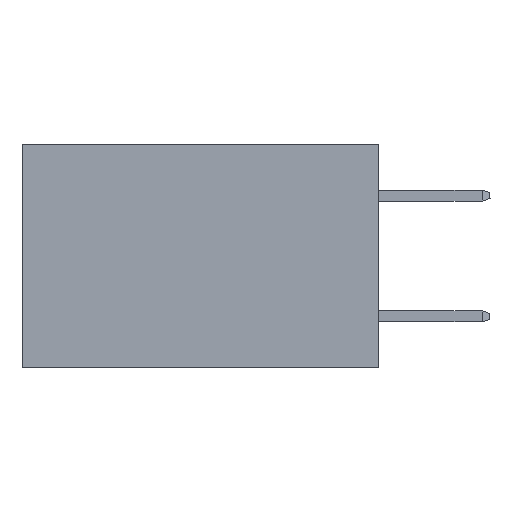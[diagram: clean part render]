
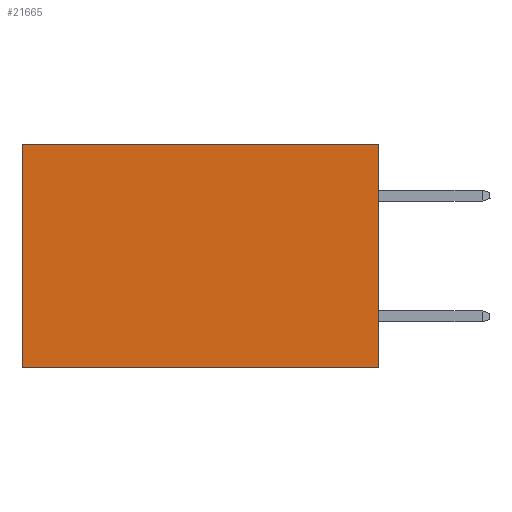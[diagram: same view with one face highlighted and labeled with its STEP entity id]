
A CAD part, left-side view. The second image highlights one B-rep face of the part: STEP entity #21665.
In plain terms, the highlighted planar face has unit normal (-1, 0, 0).
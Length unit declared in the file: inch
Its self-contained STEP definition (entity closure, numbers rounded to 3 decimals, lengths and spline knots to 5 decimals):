
#266 = VECTOR ( 'NONE', #4841, 39.37008 ) ;
#734 = AXIS2_PLACEMENT_3D ( 'NONE', #18859, #20709, #9584 ) ;
#857 = LINE ( 'NONE', #14212, #266 ) ;
#997 = CARTESIAN_POINT ( 'NONE',  ( 0.277, 0.59, 0. ) ) ;
#1750 = EDGE_CURVE ( 'NONE', #14072, #23244, #3507, .T. ) ;
#2587 = ORIENTED_EDGE ( 'NONE', *, *, #1750, .T. ) ;
#3507 = LINE ( 'NONE', #12832, #22792 ) ;
#3844 = CARTESIAN_POINT ( 'NONE',  ( 0.277, 0., -0.37 ) ) ;
#4365 = EDGE_CURVE ( 'NONE', #23244, #4594, #6956, .T. ) ;
#4594 = VERTEX_POINT ( 'NONE', #13233 ) ;
#4841 = DIRECTION ( 'NONE',  ( 0., 0., -1. ) ) ;
#6956 = LINE ( 'NONE', #18483, #21273 ) ;
#8034 = EDGE_CURVE ( 'NONE', #15046, #4594, #23812, .T. ) ;
#9166 = CARTESIAN_POINT ( 'NONE',  ( 0.277, 0., 0. ) ) ;
#9584 = DIRECTION ( 'NONE',  ( 0., 0., -1. ) ) ;
#9839 = DIRECTION ( 'NONE',  ( 0., 1., 0. ) ) ;
#11024 = FACE_OUTER_BOUND ( 'NONE', #13130, .T. ) ;
#11388 = PLANE ( 'NONE',  #734 ) ;
#12832 = CARTESIAN_POINT ( 'NONE',  ( 0.277, 0., 0. ) ) ;
#13130 = EDGE_LOOP ( 'NONE', ( #24115, #20545, #23593, #2587 ) ) ;
#13233 = CARTESIAN_POINT ( 'NONE',  ( 0.277, 0.59, -0.37 ) ) ;
#14072 = VERTEX_POINT ( 'NONE', #9166 ) ;
#14212 = CARTESIAN_POINT ( 'NONE',  ( 0.277, 0., -0.37 ) ) ;
#15046 = VERTEX_POINT ( 'NONE', #15161 ) ;
#15161 = CARTESIAN_POINT ( 'NONE',  ( 0.277, 0., -0.37 ) ) ;
#16059 = EDGE_CURVE ( 'NONE', #14072, #15046, #857, .T. ) ;
#17001 = DIRECTION ( 'NONE',  ( 0., 1., 0. ) ) ;
#18205 = DIRECTION ( 'NONE',  ( 0., 0., -1. ) ) ;
#18422 = VECTOR ( 'NONE', #17001, 39.37008 ) ;
#18483 = CARTESIAN_POINT ( 'NONE',  ( 0.277, 0.59, -0.37 ) ) ;
#18859 = CARTESIAN_POINT ( 'NONE',  ( 0.277, 0., -0.37 ) ) ;
#20545 = ORIENTED_EDGE ( 'NONE', *, *, #8034, .F. ) ;
#20709 = DIRECTION ( 'NONE',  ( 1., 0., 0. ) ) ;
#21273 = VECTOR ( 'NONE', #18205, 39.37008 ) ;
#21665 = ADVANCED_FACE ( 'NONE', ( #11024 ), #11388, .F. ) ;
#22792 = VECTOR ( 'NONE', #9839, 39.37008 ) ;
#23244 = VERTEX_POINT ( 'NONE', #997 ) ;
#23593 = ORIENTED_EDGE ( 'NONE', *, *, #16059, .F. ) ;
#23812 = LINE ( 'NONE', #3844, #18422 ) ;
#24115 = ORIENTED_EDGE ( 'NONE', *, *, #4365, .T. ) ;
